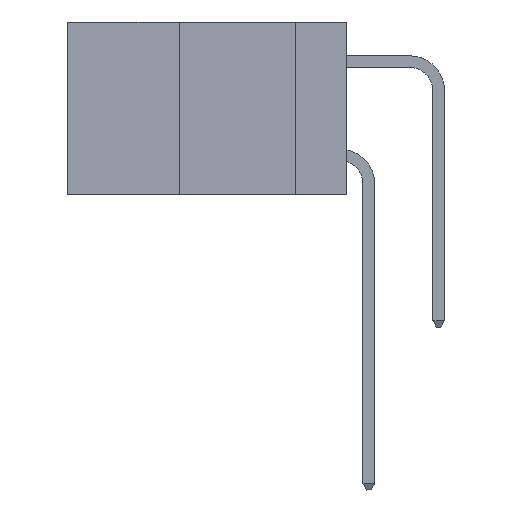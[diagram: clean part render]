
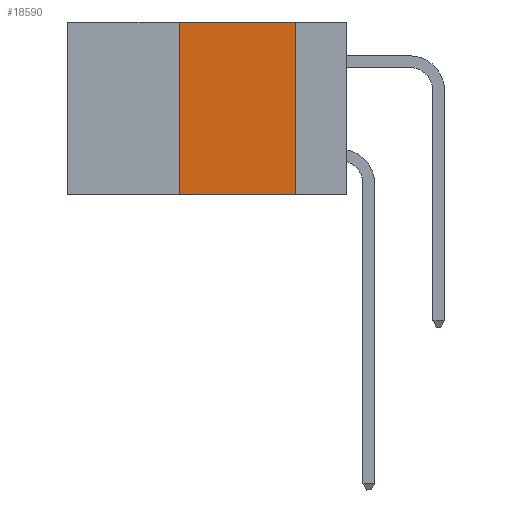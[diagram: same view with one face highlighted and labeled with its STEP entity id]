
A CAD part, left-side view. The second image highlights one B-rep face of the part: STEP entity #18590.
In plain terms, the highlighted planar face has unit normal (-1, 0, 0).
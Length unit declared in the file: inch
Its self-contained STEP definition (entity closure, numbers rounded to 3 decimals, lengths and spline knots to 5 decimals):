
#881 = ORIENTED_EDGE ( 'NONE', *, *, #6106, .F. ) ;
#1174 = PLANE ( 'NONE',  #14563 ) ;
#1444 = DIRECTION ( 'NONE',  ( 0., 0., 1. ) ) ;
#1932 = CARTESIAN_POINT ( 'NONE',  ( 0., 0.11, 0. ) ) ;
#3511 = FACE_OUTER_BOUND ( 'NONE', #3879, .T. ) ;
#3879 = EDGE_LOOP ( 'NONE', ( #26189, #12802, #881, #23342 ) ) ;
#6106 = EDGE_CURVE ( 'NONE', #23006, #26891, #9509, .T. ) ;
#8028 = EDGE_CURVE ( 'NONE', #26891, #11277, #13150, .T. ) ;
#8650 = VECTOR ( 'NONE', #1444, 39.37008 ) ;
#8895 = VECTOR ( 'NONE', #18185, 39.37008 ) ;
#9509 = LINE ( 'NONE', #30896, #8650 ) ;
#9607 = CARTESIAN_POINT ( 'NONE',  ( 0., 0.36, 0. ) ) ;
#11277 = VERTEX_POINT ( 'NONE', #1932 ) ;
#12802 = ORIENTED_EDGE ( 'NONE', *, *, #8028, .F. ) ;
#13098 = CARTESIAN_POINT ( 'NONE',  ( 0., 0.36, -0.37 ) ) ;
#13150 = LINE ( 'NONE', #18209, #19488 ) ;
#13871 = CARTESIAN_POINT ( 'NONE',  ( 0., 0.11, -0.37 ) ) ;
#14563 = AXIS2_PLACEMENT_3D ( 'NONE', #22736, #14872, #33357 ) ;
#14872 = DIRECTION ( 'NONE',  ( 1., 0., 0. ) ) ;
#15196 = EDGE_CURVE ( 'NONE', #11277, #21975, #17759, .T. ) ;
#17759 = LINE ( 'NONE', #23467, #8895 ) ;
#18185 = DIRECTION ( 'NONE',  ( 0., 0., -1. ) ) ;
#18209 = CARTESIAN_POINT ( 'NONE',  ( 0., 0.6, 0. ) ) ;
#18590 = ADVANCED_FACE ( 'NONE', ( #3511 ), #1174, .F. ) ;
#19488 = VECTOR ( 'NONE', #31368, 39.37008 ) ;
#21271 = EDGE_CURVE ( 'NONE', #23006, #21975, #27221, .T. ) ;
#21975 = VERTEX_POINT ( 'NONE', #13871 ) ;
#22736 = CARTESIAN_POINT ( 'NONE',  ( 0., 0.6, 0. ) ) ;
#23006 = VERTEX_POINT ( 'NONE', #13098 ) ;
#23342 = ORIENTED_EDGE ( 'NONE', *, *, #21271, .T. ) ;
#23467 = CARTESIAN_POINT ( 'NONE',  ( 0., 0.11, 0. ) ) ;
#26189 = ORIENTED_EDGE ( 'NONE', *, *, #15196, .F. ) ;
#26891 = VERTEX_POINT ( 'NONE', #9607 ) ;
#27221 = LINE ( 'NONE', #29680, #33322 ) ;
#29680 = CARTESIAN_POINT ( 'NONE',  ( 0., 0.6, -0.37 ) ) ;
#30896 = CARTESIAN_POINT ( 'NONE',  ( 0., 0.36, 0. ) ) ;
#31368 = DIRECTION ( 'NONE',  ( 0., -1., 0. ) ) ;
#32277 = DIRECTION ( 'NONE',  ( 0., -1., 0. ) ) ;
#33322 = VECTOR ( 'NONE', #32277, 39.37008 ) ;
#33357 = DIRECTION ( 'NONE',  ( 0., 0., -1. ) ) ;
